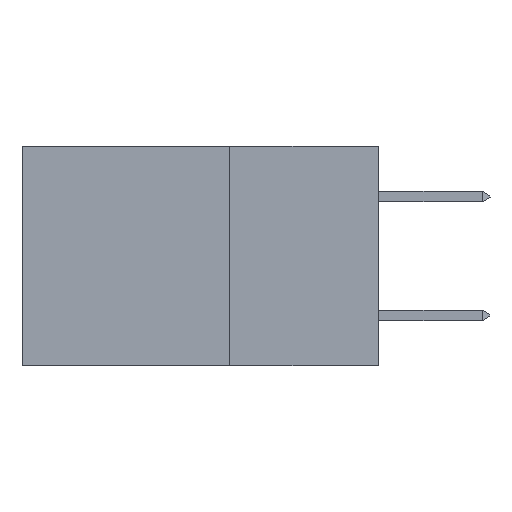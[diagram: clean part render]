
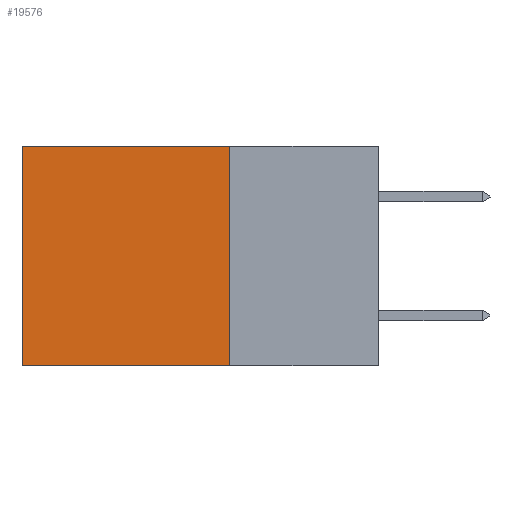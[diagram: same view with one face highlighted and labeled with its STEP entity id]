
A CAD part, left-side view. The second image highlights one B-rep face of the part: STEP entity #19576.
In plain terms, the highlighted planar face has unit normal (-1, 0, 0).
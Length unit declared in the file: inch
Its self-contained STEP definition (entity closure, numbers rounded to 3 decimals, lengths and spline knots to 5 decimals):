
#1181 = CARTESIAN_POINT ( 'NONE',  ( 0.298, 0.25, 0. ) ) ;
#1364 = PLANE ( 'NONE',  #11497 ) ;
#1441 = DIRECTION ( 'NONE',  ( 1., 0., 0. ) ) ;
#1619 = FACE_OUTER_BOUND ( 'NONE', #14748, .T. ) ;
#1984 = DIRECTION ( 'NONE',  ( 0., 0., -1. ) ) ;
#2495 = EDGE_CURVE ( 'NONE', #13695, #22791, #12557, .T. ) ;
#4200 = EDGE_CURVE ( 'NONE', #13695, #8626, #18235, .T. ) ;
#5611 = VERTEX_POINT ( 'NONE', #12201 ) ;
#5792 = EDGE_CURVE ( 'NONE', #8626, #5611, #16795, .T. ) ;
#7697 = CARTESIAN_POINT ( 'NONE',  ( 0.298, 0.25, 0. ) ) ;
#8626 = VERTEX_POINT ( 'NONE', #9269 ) ;
#9018 = LINE ( 'NONE', #21506, #17929 ) ;
#9269 = CARTESIAN_POINT ( 'NONE',  ( 0.298, 0.6, 0. ) ) ;
#10000 = ORIENTED_EDGE ( 'NONE', *, *, #2495, .F. ) ;
#10293 = CARTESIAN_POINT ( 'NONE',  ( 0.298, 0.25, 0. ) ) ;
#11497 = AXIS2_PLACEMENT_3D ( 'NONE', #10293, #1441, #13901 ) ;
#12201 = CARTESIAN_POINT ( 'NONE',  ( 0.298, 0.6, -0.37 ) ) ;
#12557 = LINE ( 'NONE', #1181, #17243 ) ;
#12662 = VECTOR ( 'NONE', #1984, 39.37008 ) ;
#12841 = DIRECTION ( 'NONE',  ( 0., 1., 0. ) ) ;
#13056 = ORIENTED_EDGE ( 'NONE', *, *, #21200, .F. ) ;
#13695 = VERTEX_POINT ( 'NONE', #15406 ) ;
#13901 = DIRECTION ( 'NONE',  ( 0., 0., -1. ) ) ;
#14446 = CARTESIAN_POINT ( 'NONE',  ( 0.298, 0.6, 0. ) ) ;
#14748 = EDGE_LOOP ( 'NONE', ( #20124, #13056, #10000, #17003 ) ) ;
#15406 = CARTESIAN_POINT ( 'NONE',  ( 0.298, 0.25, 0. ) ) ;
#16572 = DIRECTION ( 'NONE',  ( 0., 1., 0. ) ) ;
#16795 = LINE ( 'NONE', #14446, #12662 ) ;
#17003 = ORIENTED_EDGE ( 'NONE', *, *, #4200, .T. ) ;
#17243 = VECTOR ( 'NONE', #20560, 39.37008 ) ;
#17532 = CARTESIAN_POINT ( 'NONE',  ( 0.298, 0.25, -0.37 ) ) ;
#17705 = VECTOR ( 'NONE', #16572, 39.37008 ) ;
#17929 = VECTOR ( 'NONE', #12841, 39.37008 ) ;
#18235 = LINE ( 'NONE', #7697, #17705 ) ;
#19576 = ADVANCED_FACE ( 'NONE', ( #1619 ), #1364, .F. ) ;
#20124 = ORIENTED_EDGE ( 'NONE', *, *, #5792, .T. ) ;
#20560 = DIRECTION ( 'NONE',  ( 0., 0., -1. ) ) ;
#21200 = EDGE_CURVE ( 'NONE', #22791, #5611, #9018, .T. ) ;
#21506 = CARTESIAN_POINT ( 'NONE',  ( 0.298, 0.25, -0.37 ) ) ;
#22791 = VERTEX_POINT ( 'NONE', #17532 ) ;
